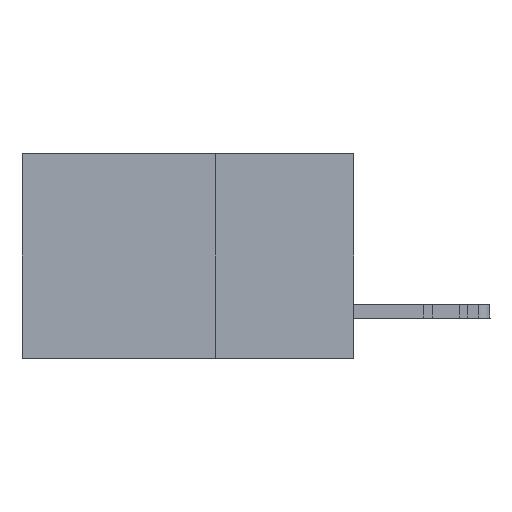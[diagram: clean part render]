
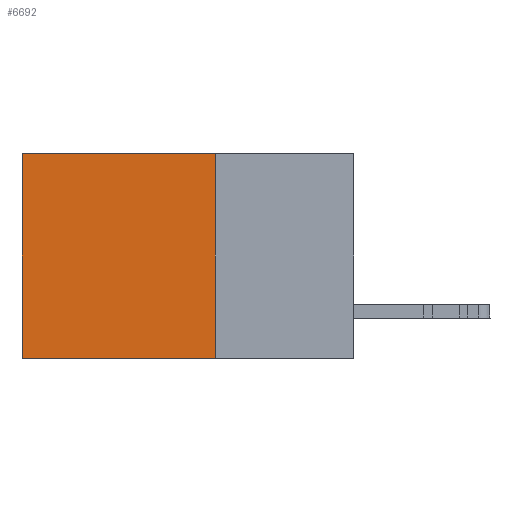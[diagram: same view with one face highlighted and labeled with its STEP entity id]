
A CAD part, left-side view. The second image highlights one B-rep face of the part: STEP entity #6692.
In plain terms, the highlighted planar face has unit normal (-1, 0, 0).
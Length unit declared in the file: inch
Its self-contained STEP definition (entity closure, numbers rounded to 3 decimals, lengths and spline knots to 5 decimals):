
#85 = LINE ( 'NONE', #3779, #32947 ) ;
#769 = CARTESIAN_POINT ( 'NONE',  ( 0.2875, 0.6, 0. ) ) ;
#2251 = CARTESIAN_POINT ( 'NONE',  ( 0.2875, 0.25, 0. ) ) ;
#2706 = ORIENTED_EDGE ( 'NONE', *, *, #4439, .F. ) ;
#3779 = CARTESIAN_POINT ( 'NONE',  ( 0.2875, 0.25, 0. ) ) ;
#4011 = FACE_OUTER_BOUND ( 'NONE', #12401, .T. ) ;
#4094 = VERTEX_POINT ( 'NONE', #25866 ) ;
#4125 = EDGE_CURVE ( 'NONE', #47736, #4094, #47780, .T. ) ;
#4439 = EDGE_CURVE ( 'NONE', #47614, #47736, #85, .T. ) ;
#6187 = DIRECTION ( 'NONE',  ( 0., 0., -1. ) ) ;
#6279 = DIRECTION ( 'NONE',  ( 0., 1., 0. ) ) ;
#6692 = ADVANCED_FACE ( 'NONE', ( #4011 ), #13730, .F. ) ;
#7274 = ORIENTED_EDGE ( 'NONE', *, *, #4125, .F. ) ;
#12401 = EDGE_LOOP ( 'NONE', ( #23271, #7274, #2706, #40820 ) ) ;
#13730 = PLANE ( 'NONE',  #20958 ) ;
#13960 = DIRECTION ( 'NONE',  ( 0., 0., -1. ) ) ;
#15097 = VERTEX_POINT ( 'NONE', #22101 ) ;
#17943 = EDGE_CURVE ( 'NONE', #47614, #15097, #47369, .T. ) ;
#20958 = AXIS2_PLACEMENT_3D ( 'NONE', #32934, #33284, #6187 ) ;
#22101 = CARTESIAN_POINT ( 'NONE',  ( 0.2875, 0.6, 0. ) ) ;
#23271 = ORIENTED_EDGE ( 'NONE', *, *, #36439, .T. ) ;
#25866 = CARTESIAN_POINT ( 'NONE',  ( 0.2875, 0.6, -0.37 ) ) ;
#25946 = DIRECTION ( 'NONE',  ( 0., 1., 0. ) ) ;
#27699 = DIRECTION ( 'NONE',  ( 0., 0., -1. ) ) ;
#31714 = VECTOR ( 'NONE', #25946, 39.37008 ) ;
#32934 = CARTESIAN_POINT ( 'NONE',  ( 0.2875, 0.25, 0. ) ) ;
#32947 = VECTOR ( 'NONE', #13960, 39.37008 ) ;
#33284 = DIRECTION ( 'NONE',  ( 1., 0., 0. ) ) ;
#35676 = VECTOR ( 'NONE', #27699, 39.37008 ) ;
#36439 = EDGE_CURVE ( 'NONE', #15097, #4094, #38151, .T. ) ;
#36787 = CARTESIAN_POINT ( 'NONE',  ( 0.2875, 0.25, -0.37 ) ) ;
#38151 = LINE ( 'NONE', #769, #35676 ) ;
#40820 = ORIENTED_EDGE ( 'NONE', *, *, #17943, .T. ) ;
#44343 = CARTESIAN_POINT ( 'NONE',  ( 0.2875, 0.25, -0.37 ) ) ;
#44857 = CARTESIAN_POINT ( 'NONE',  ( 0.2875, 0.25, 0. ) ) ;
#47369 = LINE ( 'NONE', #2251, #48707 ) ;
#47614 = VERTEX_POINT ( 'NONE', #44857 ) ;
#47736 = VERTEX_POINT ( 'NONE', #44343 ) ;
#47780 = LINE ( 'NONE', #36787, #31714 ) ;
#48707 = VECTOR ( 'NONE', #6279, 39.37008 ) ;
